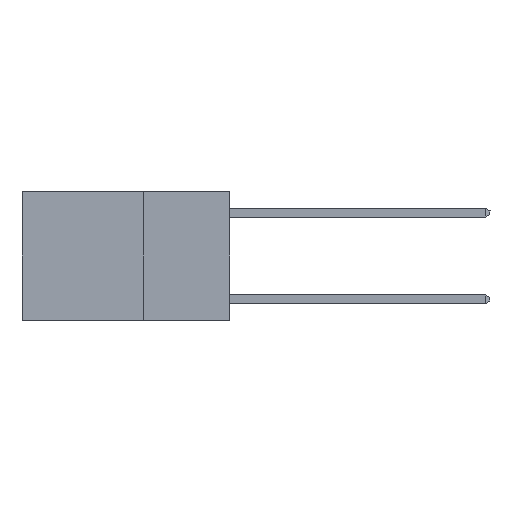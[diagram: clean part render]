
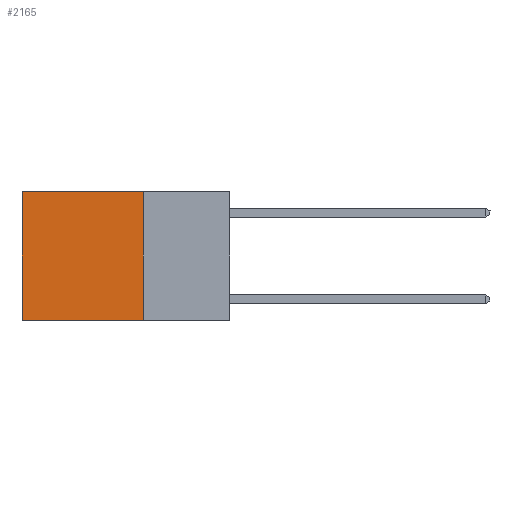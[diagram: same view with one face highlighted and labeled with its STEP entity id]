
A CAD part, left-side view. The second image highlights one B-rep face of the part: STEP entity #2165.
In plain terms, the highlighted planar face has unit normal (-1, 0, 0).
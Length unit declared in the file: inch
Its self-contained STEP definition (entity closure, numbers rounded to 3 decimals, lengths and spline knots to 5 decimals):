
#157 = VERTEX_POINT ( 'NONE', #17770 ) ;
#1532 = CARTESIAN_POINT ( 'NONE',  ( 0.2625, 0.25, -0.37 ) ) ;
#2165 = ADVANCED_FACE ( 'NONE', ( #20179 ), #13712, .F. ) ;
#3687 = CARTESIAN_POINT ( 'NONE',  ( 0.2625, 0.25, 0. ) ) ;
#4226 = LINE ( 'NONE', #21089, #16472 ) ;
#5808 = ORIENTED_EDGE ( 'NONE', *, *, #14917, .F. ) ;
#6061 = AXIS2_PLACEMENT_3D ( 'NONE', #22142, #11757, #26025 ) ;
#6332 = EDGE_CURVE ( 'NONE', #16070, #11302, #25402, .T. ) ;
#9264 = EDGE_CURVE ( 'NONE', #11302, #15608, #21665, .T. ) ;
#9598 = ORIENTED_EDGE ( 'NONE', *, *, #6332, .T. ) ;
#9629 = ORIENTED_EDGE ( 'NONE', *, *, #9264, .T. ) ;
#11302 = VERTEX_POINT ( 'NONE', #12082 ) ;
#11757 = DIRECTION ( 'NONE',  ( 1., 0., 0. ) ) ;
#12058 = LINE ( 'NONE', #1532, #23766 ) ;
#12082 = CARTESIAN_POINT ( 'NONE',  ( 0.2625, 0.6, 0. ) ) ;
#12381 = VECTOR ( 'NONE', #23743, 39.37008 ) ;
#13712 = PLANE ( 'NONE',  #6061 ) ;
#14352 = DIRECTION ( 'NONE',  ( 0., 0., -1. ) ) ;
#14646 = CARTESIAN_POINT ( 'NONE',  ( 0.2625, 0.6, -0.37 ) ) ;
#14917 = EDGE_CURVE ( 'NONE', #157, #15608, #12058, .T. ) ;
#15608 = VERTEX_POINT ( 'NONE', #14646 ) ;
#15782 = DIRECTION ( 'NONE',  ( 0., 1., 0. ) ) ;
#16070 = VERTEX_POINT ( 'NONE', #3687 ) ;
#16472 = VECTOR ( 'NONE', #14352, 39.37008 ) ;
#17245 = CARTESIAN_POINT ( 'NONE',  ( 0.2625, 0.6, 0. ) ) ;
#17770 = CARTESIAN_POINT ( 'NONE',  ( 0.2625, 0.25, -0.37 ) ) ;
#20179 = FACE_OUTER_BOUND ( 'NONE', #23690, .T. ) ;
#21089 = CARTESIAN_POINT ( 'NONE',  ( 0.2625, 0.25, 0. ) ) ;
#21236 = DIRECTION ( 'NONE',  ( 0., 1., 0. ) ) ;
#21665 = LINE ( 'NONE', #17245, #12381 ) ;
#22064 = EDGE_CURVE ( 'NONE', #16070, #157, #4226, .T. ) ;
#22142 = CARTESIAN_POINT ( 'NONE',  ( 0.2625, 0.25, 0. ) ) ;
#23639 = ORIENTED_EDGE ( 'NONE', *, *, #22064, .F. ) ;
#23690 = EDGE_LOOP ( 'NONE', ( #9629, #5808, #23639, #9598 ) ) ;
#23743 = DIRECTION ( 'NONE',  ( 0., 0., -1. ) ) ;
#23766 = VECTOR ( 'NONE', #15782, 39.37008 ) ;
#25268 = CARTESIAN_POINT ( 'NONE',  ( 0.2625, 0.25, 0. ) ) ;
#25402 = LINE ( 'NONE', #25268, #26434 ) ;
#26025 = DIRECTION ( 'NONE',  ( 0., 0., -1. ) ) ;
#26434 = VECTOR ( 'NONE', #21236, 39.37008 ) ;
